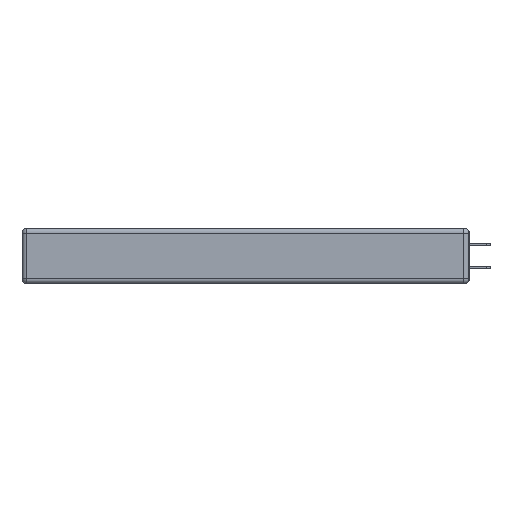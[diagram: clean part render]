
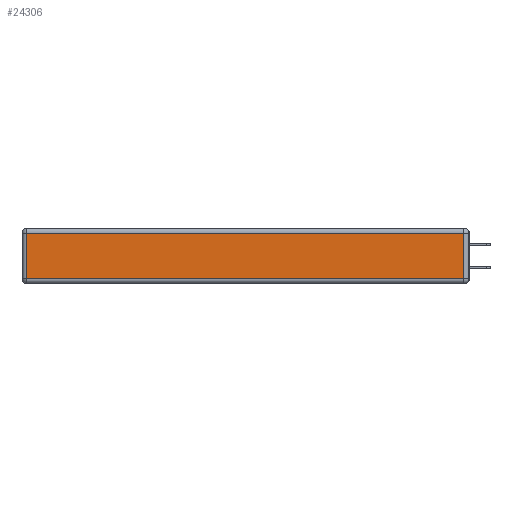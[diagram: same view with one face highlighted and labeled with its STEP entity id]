
A CAD part, left-side view. The second image highlights one B-rep face of the part: STEP entity #24306.
In plain terms, the highlighted planar face has unit normal (-1, 0, 0).
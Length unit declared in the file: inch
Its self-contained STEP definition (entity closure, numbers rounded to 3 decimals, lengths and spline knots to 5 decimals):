
#284 = ORIENTED_EDGE ( 'NONE', *, *, #286, .T. ) ;
#286 = EDGE_CURVE ( 'NONE', #20715, #5790, #6621, .T. ) ;
#335 = CARTESIAN_POINT ( 'NONE',  ( 0., 2.75, -0.03 ) ) ;
#1325 = DIRECTION ( 'NONE',  ( 0., 0., 1. ) ) ;
#2053 = CARTESIAN_POINT ( 'NONE',  ( 0., 0.03, -0.313 ) ) ;
#4298 = DIRECTION ( 'NONE',  ( 0., 0., 1. ) ) ;
#4820 = LINE ( 'NONE', #335, #24737 ) ;
#5034 = VERTEX_POINT ( 'NONE', #15359 ) ;
#5790 = VERTEX_POINT ( 'NONE', #2053 ) ;
#5916 = VECTOR ( 'NONE', #4298, 39.37008 ) ;
#6146 = CARTESIAN_POINT ( 'NONE',  ( 0., 0.03, -0.03 ) ) ;
#6621 = LINE ( 'NONE', #7628, #6920 ) ;
#6867 = EDGE_CURVE ( 'NONE', #5790, #24534, #17668, .T. ) ;
#6920 = VECTOR ( 'NONE', #22838, 39.37008 ) ;
#7628 = CARTESIAN_POINT ( 'NONE',  ( 0., 0., -0.313 ) ) ;
#8691 = PLANE ( 'NONE',  #11925 ) ;
#8848 = DIRECTION ( 'NONE',  ( -1., 0., 0. ) ) ;
#9488 = ORIENTED_EDGE ( 'NONE', *, *, #6867, .T. ) ;
#9926 = DIRECTION ( 'NONE',  ( 0., 0., -1. ) ) ;
#10004 = CARTESIAN_POINT ( 'NONE',  ( 0., 0.03, -0.343 ) ) ;
#11925 = AXIS2_PLACEMENT_3D ( 'NONE', #20450, #8848, #1325 ) ;
#12512 = EDGE_CURVE ( 'NONE', #5034, #20715, #20603, .T. ) ;
#15353 = FACE_OUTER_BOUND ( 'NONE', #23723, .T. ) ;
#15359 = CARTESIAN_POINT ( 'NONE',  ( 0., 2.72, -0.03 ) ) ;
#15637 = CARTESIAN_POINT ( 'NONE',  ( 0., 2.72, -0.313 ) ) ;
#16327 = EDGE_CURVE ( 'NONE', #24534, #5034, #4820, .T. ) ;
#17279 = DIRECTION ( 'NONE',  ( 0., 1., 0. ) ) ;
#17572 = VECTOR ( 'NONE', #9926, 39.37008 ) ;
#17668 = LINE ( 'NONE', #10004, #5916 ) ;
#19575 = ORIENTED_EDGE ( 'NONE', *, *, #16327, .T. ) ;
#20450 = CARTESIAN_POINT ( 'NONE',  ( 0., 0., -0.343 ) ) ;
#20603 = LINE ( 'NONE', #21536, #17572 ) ;
#20715 = VERTEX_POINT ( 'NONE', #15637 ) ;
#21536 = CARTESIAN_POINT ( 'NONE',  ( 0., 2.72, -0.343 ) ) ;
#22838 = DIRECTION ( 'NONE',  ( 0., -1., 0. ) ) ;
#23438 = ORIENTED_EDGE ( 'NONE', *, *, #12512, .T. ) ;
#23723 = EDGE_LOOP ( 'NONE', ( #284, #9488, #19575, #23438 ) ) ;
#24306 = ADVANCED_FACE ( 'NONE', ( #15353 ), #8691, .T. ) ;
#24534 = VERTEX_POINT ( 'NONE', #6146 ) ;
#24737 = VECTOR ( 'NONE', #17279, 39.37008 ) ;
